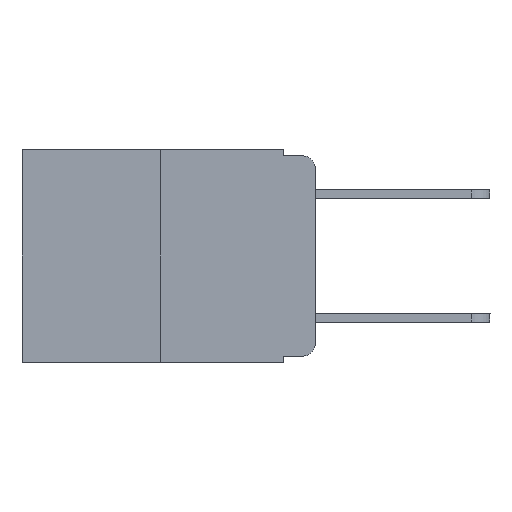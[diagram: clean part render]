
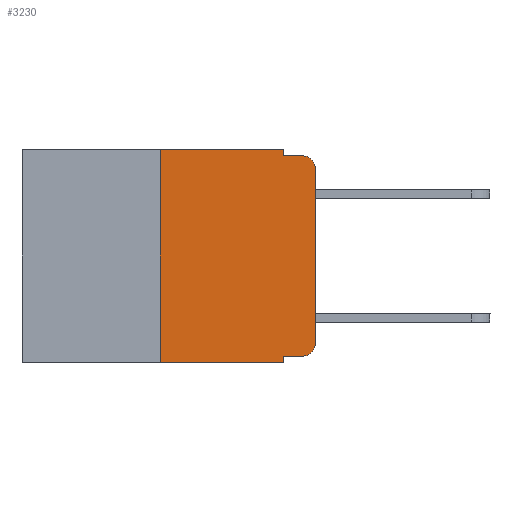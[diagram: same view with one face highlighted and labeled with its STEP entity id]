
A CAD part, left-side view. The second image highlights one B-rep face of the part: STEP entity #3230.
In plain terms, the highlighted planar face has unit normal (-1, 0, 0).
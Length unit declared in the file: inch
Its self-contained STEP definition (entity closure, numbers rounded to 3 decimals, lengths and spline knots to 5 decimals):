
#566 = VERTEX_POINT ( 'NONE', #15417 ) ;
#890 = DIRECTION ( 'NONE',  ( -1., 0., 0. ) ) ;
#1466 = CARTESIAN_POINT ( 'NONE',  ( 0., 0.02, -0.03 ) ) ;
#1549 = VERTEX_POINT ( 'NONE', #24568 ) ;
#1988 = CARTESIAN_POINT ( 'NONE',  ( 0., 0.051, -0.01 ) ) ;
#2138 = DIRECTION ( 'NONE',  ( 0., 0., 1. ) ) ;
#2411 = ORIENTED_EDGE ( 'NONE', *, *, #14996, .T. ) ;
#2625 = EDGE_CURVE ( 'NONE', #27018, #22262, #22739, .T. ) ;
#2815 = LINE ( 'NONE', #6245, #22760 ) ;
#3028 = LINE ( 'NONE', #13052, #9213 ) ;
#3230 = ADVANCED_FACE ( 'NONE', ( #24352 ), #25747, .F. ) ;
#3255 = ORIENTED_EDGE ( 'NONE', *, *, #10692, .T. ) ;
#4620 = CARTESIAN_POINT ( 'NONE',  ( 0., 0.051, 0. ) ) ;
#4624 = EDGE_LOOP ( 'NONE', ( #25730, #3255, #22240, #23688, #20089, #14711, #2411, #24758, #15713, #17537 ) ) ;
#4795 = CIRCLE ( 'NONE', #26250, 0.02 ) ;
#5237 = CARTESIAN_POINT ( 'NONE',  ( 0., 0.02, -0.333 ) ) ;
#5264 = CARTESIAN_POINT ( 'NONE',  ( 0., 0.02, -0.01 ) ) ;
#5647 = DIRECTION ( 'NONE',  ( 0., 0., -1. ) ) ;
#5774 = VERTEX_POINT ( 'NONE', #19766 ) ;
#6048 = LINE ( 'NONE', #1988, #10934 ) ;
#6245 = CARTESIAN_POINT ( 'NONE',  ( 0., 0., 0. ) ) ;
#6740 = DIRECTION ( 'NONE',  ( 0., 0., -1. ) ) ;
#6896 = CARTESIAN_POINT ( 'NONE',  ( 0., 0.02, -0.313 ) ) ;
#7006 = CARTESIAN_POINT ( 'NONE',  ( 0., 0., -0.03 ) ) ;
#7398 = VERTEX_POINT ( 'NONE', #5264 ) ;
#7711 = CARTESIAN_POINT ( 'NONE',  ( 0., 0.051, -0.333 ) ) ;
#8194 = CARTESIAN_POINT ( 'NONE',  ( 0., 0.051, -0.01 ) ) ;
#8218 = DIRECTION ( 'NONE',  ( 0., -1., 0. ) ) ;
#8603 = VECTOR ( 'NONE', #8218, 39.37008 ) ;
#8868 = LINE ( 'NONE', #24652, #24888 ) ;
#9213 = VECTOR ( 'NONE', #13313, 39.37008 ) ;
#9451 = VERTEX_POINT ( 'NONE', #7006 ) ;
#9778 = CARTESIAN_POINT ( 'NONE',  ( 0., 0.25, 0. ) ) ;
#10663 = VERTEX_POINT ( 'NONE', #19982 ) ;
#10692 = EDGE_CURVE ( 'NONE', #9451, #7398, #4795, .T. ) ;
#10934 = VECTOR ( 'NONE', #18581, 39.37008 ) ;
#11760 = AXIS2_PLACEMENT_3D ( 'NONE', #23570, #23655, #6740 ) ;
#12205 = EDGE_CURVE ( 'NONE', #15224, #7398, #6048, .T. ) ;
#12798 = LINE ( 'NONE', #9778, #13435 ) ;
#13052 = CARTESIAN_POINT ( 'NONE',  ( 0., 0.051, 0. ) ) ;
#13313 = DIRECTION ( 'NONE',  ( 0., 0., -1. ) ) ;
#13435 = VECTOR ( 'NONE', #22378, 39.37008 ) ;
#13471 = CARTESIAN_POINT ( 'NONE',  ( 0., 0.473, -0.343 ) ) ;
#14135 = DIRECTION ( 'NONE',  ( -1., 0., 0. ) ) ;
#14290 = EDGE_CURVE ( 'NONE', #27018, #566, #3028, .T. ) ;
#14298 = DIRECTION ( 'NONE',  ( 0., 0., -1. ) ) ;
#14711 = ORIENTED_EDGE ( 'NONE', *, *, #17668, .F. ) ;
#14746 = CARTESIAN_POINT ( 'NONE',  ( 0., 0.051, -0.333 ) ) ;
#14996 = EDGE_CURVE ( 'NONE', #5774, #566, #22275, .T. ) ;
#15224 = VERTEX_POINT ( 'NONE', #8194 ) ;
#15417 = CARTESIAN_POINT ( 'NONE',  ( 0., 0.051, -0.343 ) ) ;
#15492 = EDGE_CURVE ( 'NONE', #22262, #10663, #22573, .T. ) ;
#15537 = DIRECTION ( 'NONE',  ( 0., 0., -1. ) ) ;
#15713 = ORIENTED_EDGE ( 'NONE', *, *, #2625, .T. ) ;
#16145 = VERTEX_POINT ( 'NONE', #4620 ) ;
#17537 = ORIENTED_EDGE ( 'NONE', *, *, #15492, .T. ) ;
#17668 = EDGE_CURVE ( 'NONE', #5774, #1549, #12798, .T. ) ;
#18581 = DIRECTION ( 'NONE',  ( 0., -1., 0. ) ) ;
#19766 = CARTESIAN_POINT ( 'NONE',  ( 0., 0.25, -0.343 ) ) ;
#19779 = VECTOR ( 'NONE', #20500, 39.37008 ) ;
#19982 = CARTESIAN_POINT ( 'NONE',  ( 0., 0., -0.313 ) ) ;
#20089 = ORIENTED_EDGE ( 'NONE', *, *, #24960, .F. ) ;
#20500 = DIRECTION ( 'NONE',  ( 0., -1., 0. ) ) ;
#20917 = EDGE_CURVE ( 'NONE', #10663, #9451, #2815, .T. ) ;
#20975 = VECTOR ( 'NONE', #21999, 39.37008 ) ;
#21999 = DIRECTION ( 'NONE',  ( 0., -1., 0. ) ) ;
#22240 = ORIENTED_EDGE ( 'NONE', *, *, #12205, .F. ) ;
#22262 = VERTEX_POINT ( 'NONE', #5237 ) ;
#22275 = LINE ( 'NONE', #13471, #20975 ) ;
#22378 = DIRECTION ( 'NONE',  ( 0., 0., 1. ) ) ;
#22573 = CIRCLE ( 'NONE', #23189, 0.02 ) ;
#22739 = LINE ( 'NONE', #7711, #19779 ) ;
#22760 = VECTOR ( 'NONE', #2138, 39.37008 ) ;
#22942 = CARTESIAN_POINT ( 'NONE',  ( 0., 0.473, 0. ) ) ;
#23189 = AXIS2_PLACEMENT_3D ( 'NONE', #6896, #890, #15537 ) ;
#23570 = CARTESIAN_POINT ( 'NONE',  ( 0., 0.473, 0. ) ) ;
#23655 = DIRECTION ( 'NONE',  ( 1., 0., 0. ) ) ;
#23688 = ORIENTED_EDGE ( 'NONE', *, *, #26914, .F. ) ;
#24352 = FACE_OUTER_BOUND ( 'NONE', #4624, .T. ) ;
#24568 = CARTESIAN_POINT ( 'NONE',  ( 0., 0.25, 0. ) ) ;
#24652 = CARTESIAN_POINT ( 'NONE',  ( 0., 0.051, 0. ) ) ;
#24758 = ORIENTED_EDGE ( 'NONE', *, *, #14290, .F. ) ;
#24888 = VECTOR ( 'NONE', #14298, 39.37008 ) ;
#24957 = LINE ( 'NONE', #22942, #8603 ) ;
#24960 = EDGE_CURVE ( 'NONE', #1549, #16145, #24957, .T. ) ;
#25730 = ORIENTED_EDGE ( 'NONE', *, *, #20917, .T. ) ;
#25747 = PLANE ( 'NONE',  #11760 ) ;
#26250 = AXIS2_PLACEMENT_3D ( 'NONE', #1466, #14135, #5647 ) ;
#26914 = EDGE_CURVE ( 'NONE', #16145, #15224, #8868, .T. ) ;
#27018 = VERTEX_POINT ( 'NONE', #14746 ) ;
